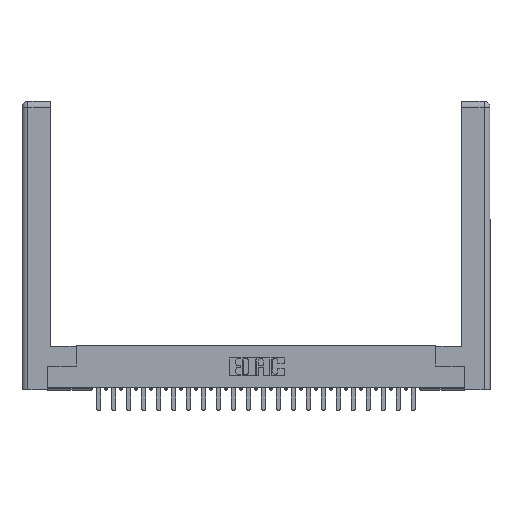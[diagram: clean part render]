
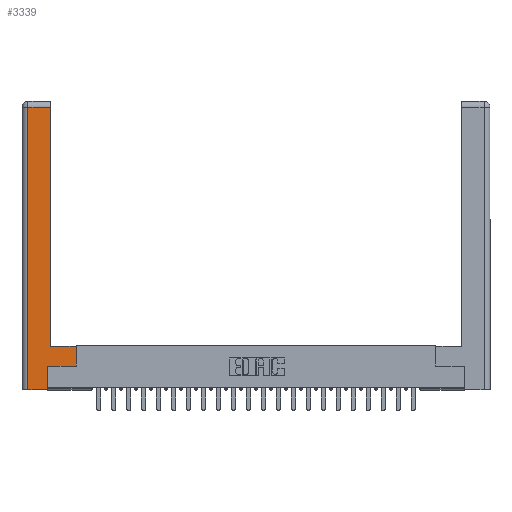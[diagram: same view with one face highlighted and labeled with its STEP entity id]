
A CAD part, top view. The second image highlights one B-rep face of the part: STEP entity #3339.
In plain terms, the highlighted planar face has unit normal (0, 0, 1).
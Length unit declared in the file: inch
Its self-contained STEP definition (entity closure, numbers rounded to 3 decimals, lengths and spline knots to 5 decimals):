
#513 = CARTESIAN_POINT ( 'NONE',  ( 0.295, 2.94, 0. ) ) ;
#761 = DIRECTION ( 'NONE',  ( 0., 1., 0. ) ) ;
#837 = ORIENTED_EDGE ( 'NONE', *, *, #27988, .T. ) ;
#1918 = CARTESIAN_POINT ( 'NONE',  ( 0.0615, 0., 0. ) ) ;
#2095 = DIRECTION ( 'NONE',  ( 0., 1., 0. ) ) ;
#2099 = VERTEX_POINT ( 'NONE', #12667 ) ;
#2373 = VECTOR ( 'NONE', #2095, 39.37008 ) ;
#3215 = EDGE_CURVE ( 'NONE', #22505, #18413, #5378, .T. ) ;
#3339 = ADVANCED_FACE ( 'NONE', ( #16118 ), #18365, .F. ) ;
#3995 = DIRECTION ( 'NONE',  ( -1., 0., 0. ) ) ;
#4243 = CARTESIAN_POINT ( 'NONE',  ( 0.265, 0., 0. ) ) ;
#4283 = ORIENTED_EDGE ( 'NONE', *, *, #13308, .T. ) ;
#4302 = CARTESIAN_POINT ( 'NONE',  ( 0.565, 0.245, 0. ) ) ;
#4741 = AXIS2_PLACEMENT_3D ( 'NONE', #20585, #7203, #7490 ) ;
#4771 = CARTESIAN_POINT ( 'NONE',  ( 0.265, 0.245, 0. ) ) ;
#5378 = LINE ( 'NONE', #21809, #8153 ) ;
#6120 = CARTESIAN_POINT ( 'NONE',  ( 0.0615, 2.94, 0. ) ) ;
#6698 = ORIENTED_EDGE ( 'NONE', *, *, #8985, .T. ) ;
#7203 = DIRECTION ( 'NONE',  ( 0., 0., -1. ) ) ;
#7490 = DIRECTION ( 'NONE',  ( -1., 0., 0. ) ) ;
#7690 = DIRECTION ( 'NONE',  ( -1., 0., 0. ) ) ;
#7886 = CARTESIAN_POINT ( 'NONE',  ( 0.295, 0.45, 0. ) ) ;
#8153 = VECTOR ( 'NONE', #26285, 39.37008 ) ;
#8985 = EDGE_CURVE ( 'NONE', #16467, #19506, #11755, .T. ) ;
#10194 = CARTESIAN_POINT ( 'NONE',  ( 0.0615, 2.94, 0. ) ) ;
#10286 = VECTOR ( 'NONE', #19819, 39.37008 ) ;
#10360 = ORIENTED_EDGE ( 'NONE', *, *, #3215, .T. ) ;
#10439 = EDGE_CURVE ( 'NONE', #2099, #27909, #15810, .T. ) ;
#10686 = VERTEX_POINT ( 'NONE', #12006 ) ;
#11194 = ORIENTED_EDGE ( 'NONE', *, *, #10439, .T. ) ;
#11331 = LINE ( 'NONE', #4302, #10286 ) ;
#11386 = ORIENTED_EDGE ( 'NONE', *, *, #20208, .T. ) ;
#11755 = LINE ( 'NONE', #17806, #2373 ) ;
#12006 = CARTESIAN_POINT ( 'NONE',  ( 0.265, 0.245, 0. ) ) ;
#12031 = LINE ( 'NONE', #6120, #23137 ) ;
#12155 = CARTESIAN_POINT ( 'NONE',  ( 0.565, 0.245, 0. ) ) ;
#12351 = LINE ( 'NONE', #7886, #24870 ) ;
#12667 = CARTESIAN_POINT ( 'NONE',  ( 0.295, 0.45, 0. ) ) ;
#12800 = LINE ( 'NONE', #1918, #15923 ) ;
#13049 = LINE ( 'NONE', #4771, #19646 ) ;
#13308 = EDGE_CURVE ( 'NONE', #27909, #15904, #12031, .T. ) ;
#15696 = ORIENTED_EDGE ( 'NONE', *, *, #25542, .T. ) ;
#15810 = LINE ( 'NONE', #27270, #16518 ) ;
#15832 = DIRECTION ( 'NONE',  ( 0., 1., 0. ) ) ;
#15904 = VERTEX_POINT ( 'NONE', #10194 ) ;
#15923 = VECTOR ( 'NONE', #24143, 39.37008 ) ;
#16118 = FACE_OUTER_BOUND ( 'NONE', #25245, .T. ) ;
#16467 = VERTEX_POINT ( 'NONE', #12155 ) ;
#16518 = VECTOR ( 'NONE', #761, 39.37008 ) ;
#17542 = CARTESIAN_POINT ( 'NONE',  ( 0.565, 0.45, 0. ) ) ;
#17806 = CARTESIAN_POINT ( 'NONE',  ( 0.565, 0.45, 0. ) ) ;
#18365 = PLANE ( 'NONE',  #4741 ) ;
#18413 = VERTEX_POINT ( 'NONE', #4243 ) ;
#19506 = VERTEX_POINT ( 'NONE', #17542 ) ;
#19646 = VECTOR ( 'NONE', #15832, 39.37008 ) ;
#19819 = DIRECTION ( 'NONE',  ( 1., 0., 0. ) ) ;
#20036 = ORIENTED_EDGE ( 'NONE', *, *, #27331, .T. ) ;
#20208 = EDGE_CURVE ( 'NONE', #10686, #16467, #11331, .T. ) ;
#20585 = CARTESIAN_POINT ( 'NONE',  ( 0., 0., 0. ) ) ;
#21809 = CARTESIAN_POINT ( 'NONE',  ( 0.265, 0., 0. ) ) ;
#22505 = VERTEX_POINT ( 'NONE', #27687 ) ;
#23137 = VECTOR ( 'NONE', #3995, 39.37008 ) ;
#24143 = DIRECTION ( 'NONE',  ( 0., -1., 0. ) ) ;
#24870 = VECTOR ( 'NONE', #7690, 39.37008 ) ;
#25245 = EDGE_LOOP ( 'NONE', ( #11194, #4283, #15696, #10360, #20036, #11386, #6698, #837 ) ) ;
#25542 = EDGE_CURVE ( 'NONE', #15904, #22505, #12800, .T. ) ;
#26285 = DIRECTION ( 'NONE',  ( 1., 0., 0. ) ) ;
#27270 = CARTESIAN_POINT ( 'NONE',  ( 0.295, 3., 0. ) ) ;
#27331 = EDGE_CURVE ( 'NONE', #18413, #10686, #13049, .T. ) ;
#27687 = CARTESIAN_POINT ( 'NONE',  ( 0.0615, 0., 0. ) ) ;
#27909 = VERTEX_POINT ( 'NONE', #513 ) ;
#27988 = EDGE_CURVE ( 'NONE', #19506, #2099, #12351, .T. ) ;
